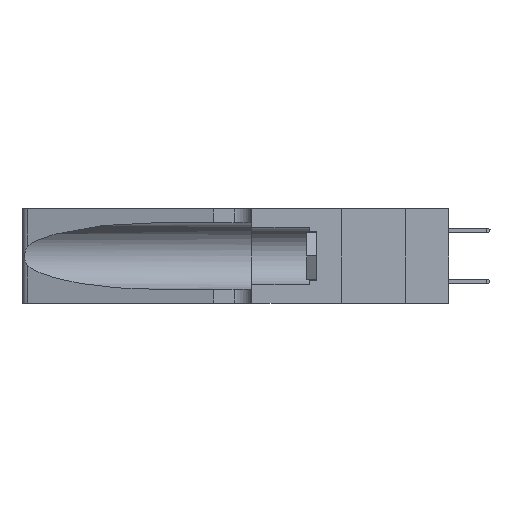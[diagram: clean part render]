
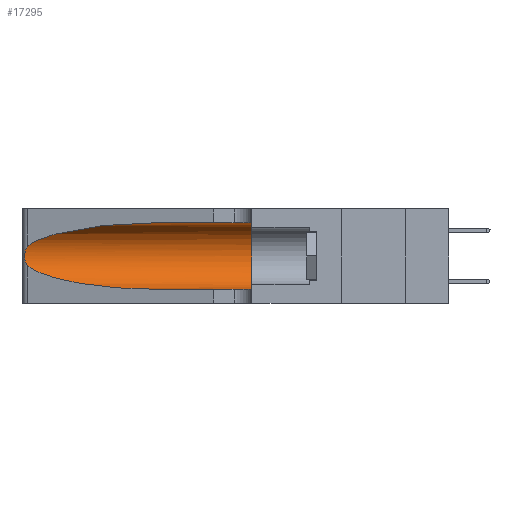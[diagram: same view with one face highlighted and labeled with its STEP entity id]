
A CAD part, left-side view. The second image highlights one B-rep face of the part: STEP entity #17295.
In plain terms, the highlighted cylindrical face has radius 3.308 mm (diameter 6.617 mm), a partial arc.
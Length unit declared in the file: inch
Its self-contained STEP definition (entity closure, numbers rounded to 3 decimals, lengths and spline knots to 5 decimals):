
#572 = CARTESIAN_POINT ( 'NONE',  ( 0.1305, 0.35, 0.05475 ) ) ;
#1323 = AXIS2_PLACEMENT_3D ( 'NONE', #40465, #6239, #40952 ) ;
#1406 = CARTESIAN_POINT ( 'NONE',  ( 0.1305, 0.72297, 0.05475 ) ) ;
#2715 = EDGE_LOOP ( 'NONE', ( #20089, #6426, #27698, #13626, #36882, #29455 ) ) ;
#3198 = CARTESIAN_POINT ( 'NONE',  ( 0.25487, 1.22718, 0.14631 ) ) ;
#3798 = EDGE_CURVE ( 'NONE', #36210, #15195, #23003, .T. ) ;
#4048 = CARTESIAN_POINT ( 'NONE',  ( 0.1305, 1.61858, 0.185 ) ) ;
#4515 = LINE ( 'NONE', #43235, #32260 ) ;
#5398 = EDGE_CURVE ( 'NONE', #22956, #35926, #36562, .T. ) ;
#6239 = DIRECTION ( 'NONE',  ( 0., 1., 0. ) ) ;
#6426 = ORIENTED_EDGE ( 'NONE', *, *, #12256, .T. ) ;
#6954 = EDGE_CURVE ( 'NONE', #15195, #41892, #27344, .T. ) ;
#8364 = CYLINDRICAL_SURFACE ( 'NONE', #26362, 0.13025 ) ;
#8684 = DIRECTION ( 'NONE',  ( 0., -1., 0. ) ) ;
#9143 = CARTESIAN_POINT ( 'NONE',  ( 0.25487, 1.22718, 0.22369 ) ) ;
#9650 = CARTESIAN_POINT ( 'NONE',  ( 0.18966, 0.96281, 0.31525 ) ) ;
#9902 = CARTESIAN_POINT ( 'NONE',  ( 0.25789, 1.23486, 0.15765 ) ) ;
#12256 = EDGE_CURVE ( 'NONE', #35926, #36210, #32399, .T. ) ;
#13574 = EDGE_CURVE ( 'NONE', #22956, #40848, #4515, .T. ) ;
#13584 = CARTESIAN_POINT ( 'NONE',  ( 0.25639, 1.23184, 0.21858 ) ) ;
#13626 = ORIENTED_EDGE ( 'NONE', *, *, #6954, .T. ) ;
#14422 = DIRECTION ( 'NONE',  ( 0., -1., 0. ) ) ;
#15195 = VERTEX_POINT ( 'NONE', #1406 ) ;
#16775 = CARTESIAN_POINT ( 'NONE',  ( 0.26075, 1.23896, 0.19203 ) ) ;
#17295 = ADVANCED_FACE ( 'NONE', ( #17651 ), #8364, .F. ) ;
#17651 = FACE_OUTER_BOUND ( 'NONE', #2715, .T. ) ;
#18025 = VECTOR ( 'NONE', #38253, 39.37008 ) ;
#18648 = DIRECTION ( 'NONE',  ( 0., 0., -1. ) ) ;
#20027 = CARTESIAN_POINT ( 'NONE',  ( 0.25487, 1.22718, 0.22369 ) ) ;
#20089 = ORIENTED_EDGE ( 'NONE', *, *, #5398, .T. ) ;
#20189 = CIRCLE ( 'NONE', #1323, 0.13025 ) ;
#20295 = CARTESIAN_POINT ( 'NONE',  ( 0.26017, 1.23833, 0.17102 ) ) ;
#20730 = CARTESIAN_POINT ( 'NONE',  ( 0.25555, 1.22994, 0.2215 ) ) ;
#20846 = CARTESIAN_POINT ( 'NONE',  ( 0.18966, 0.96281, 0.05475 ) ) ;
#20877 = CARTESIAN_POINT ( 'NONE',  ( 0.25787, 1.23484, 0.2124 ) ) ;
#22724 = CARTESIAN_POINT ( 'NONE',  ( 0.25487, 1.22718, 0.14631 ) ) ;
#22956 = VERTEX_POINT ( 'NONE', #33547 ) ;
#23003 =( BOUNDED_CURVE ( )  B_SPLINE_CURVE ( 3, ( #22724, #23152, #20846, #25513 ),
 .UNSPECIFIED., .F., .F. ) 
 B_SPLINE_CURVE_WITH_KNOTS ( ( 4, 4 ),
 ( 3.44316, 4.71239 ),
 .UNSPECIFIED. ) 
 CURVE ( )  GEOMETRIC_REPRESENTATION_ITEM ( )  RATIONAL_B_SPLINE_CURVE ( ( 1., 0.87, 0.87, 1. ) ) 
 REPRESENTATION_ITEM ( '' )  );
#23152 = CARTESIAN_POINT ( 'NONE',  ( 0.2373, 1.15595, 0.08982 ) ) ;
#23391 = CARTESIAN_POINT ( 'NONE',  ( 0.1305, 0.72297, 0.31525 ) ) ;
#24084 = CARTESIAN_POINT ( 'NONE',  ( 0.26018, 1.23835, 0.19895 ) ) ;
#25513 = CARTESIAN_POINT ( 'NONE',  ( 0.1305, 0.72297, 0.05475 ) ) ;
#26362 = AXIS2_PLACEMENT_3D ( 'NONE', #4048, #14422, #18648 ) ;
#27311 = CARTESIAN_POINT ( 'NONE',  ( 0.25856, 1.23593, 0.16098 ) ) ;
#27344 = LINE ( 'NONE', #34745, #18025 ) ;
#27468 = CARTESIAN_POINT ( 'NONE',  ( 0.25639, 1.23186, 0.15144 ) ) ;
#27698 = ORIENTED_EDGE ( 'NONE', *, *, #3798, .T. ) ;
#29371 = EDGE_CURVE ( 'NONE', #40848, #41892, #20189, .T. ) ;
#29455 = ORIENTED_EDGE ( 'NONE', *, *, #13574, .F. ) ;
#32260 = VECTOR ( 'NONE', #8684, 39.37008 ) ;
#32399 = B_SPLINE_CURVE_WITH_KNOTS ( 'NONE', 3,
 ( #34811, #20730, #13584, #20877, #37893, #24084, #16775, #41092, #20295, #27311, #9902, #27468, #34227, #3198 ),
 .UNSPECIFIED., .F., .F.,
 ( 4, 2, 2, 2, 2, 2, 4 ),
 ( 0., 0.00027, 0.00053, 0.00107, 0.0016, 0.00187, 0.00214 ),
 .UNSPECIFIED. ) ;
#33547 = CARTESIAN_POINT ( 'NONE',  ( 0.1305, 0.72297, 0.31525 ) ) ;
#34054 = CARTESIAN_POINT ( 'NONE',  ( 0.1305, 0.35, 0.31525 ) ) ;
#34227 = CARTESIAN_POINT ( 'NONE',  ( 0.25555, 1.22993, 0.14849 ) ) ;
#34745 = CARTESIAN_POINT ( 'NONE',  ( 0.1305, 1.61858, 0.05475 ) ) ;
#34811 = CARTESIAN_POINT ( 'NONE',  ( 0.25487, 1.22718, 0.22369 ) ) ;
#35926 = VERTEX_POINT ( 'NONE', #9143 ) ;
#36210 = VERTEX_POINT ( 'NONE', #45032 ) ;
#36562 =( BOUNDED_CURVE ( )  B_SPLINE_CURVE ( 3, ( #23391, #9650, #37461, #20027 ),
 .UNSPECIFIED., .F., .F. ) 
 B_SPLINE_CURVE_WITH_KNOTS ( ( 4, 4 ),
 ( 1.5708, 2.84003 ),
 .UNSPECIFIED. ) 
 CURVE ( )  GEOMETRIC_REPRESENTATION_ITEM ( )  RATIONAL_B_SPLINE_CURVE ( ( 1., 0.87, 0.87, 1. ) ) 
 REPRESENTATION_ITEM ( '' )  );
#36882 = ORIENTED_EDGE ( 'NONE', *, *, #29371, .F. ) ;
#37461 = CARTESIAN_POINT ( 'NONE',  ( 0.2373, 1.15595, 0.28018 ) ) ;
#37893 = CARTESIAN_POINT ( 'NONE',  ( 0.25854, 1.2359, 0.20912 ) ) ;
#38253 = DIRECTION ( 'NONE',  ( 0., -1., 0. ) ) ;
#40465 = CARTESIAN_POINT ( 'NONE',  ( 0.1305, 0.35, 0.185 ) ) ;
#40848 = VERTEX_POINT ( 'NONE', #34054 ) ;
#40952 = DIRECTION ( 'NONE',  ( 0., 0., 1. ) ) ;
#41092 = CARTESIAN_POINT ( 'NONE',  ( 0.26075, 1.23896, 0.178 ) ) ;
#41892 = VERTEX_POINT ( 'NONE', #572 ) ;
#43235 = CARTESIAN_POINT ( 'NONE',  ( 0.1305, 1.61858, 0.31525 ) ) ;
#45032 = CARTESIAN_POINT ( 'NONE',  ( 0.25487, 1.22718, 0.14631 ) ) ;
